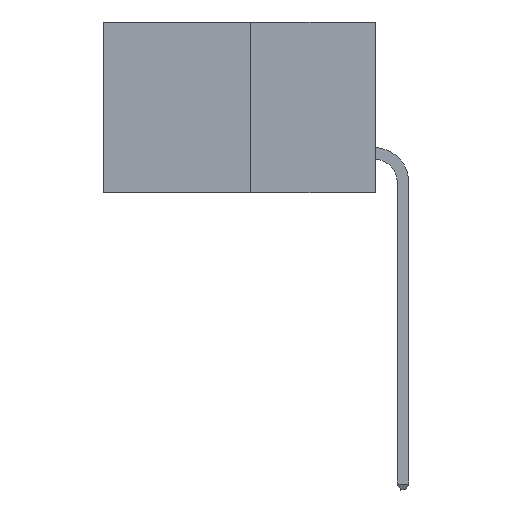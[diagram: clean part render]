
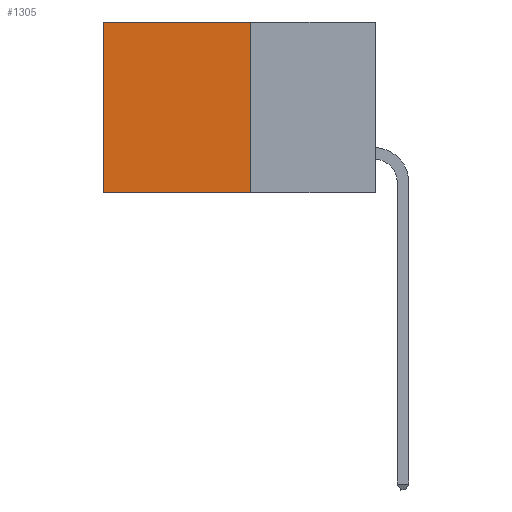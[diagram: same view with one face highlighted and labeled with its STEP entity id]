
A CAD part, left-side view. The second image highlights one B-rep face of the part: STEP entity #1305.
In plain terms, the highlighted planar face has unit normal (-1, 0, 0).
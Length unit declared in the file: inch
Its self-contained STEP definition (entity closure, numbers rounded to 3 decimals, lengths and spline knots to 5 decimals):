
#462 = DIRECTION ( 'NONE',  ( 0., 0., -1. ) ) ;
#862 = CARTESIAN_POINT ( 'NONE',  ( 0.277, 0.59, -0.37 ) ) ;
#1059 = DIRECTION ( 'NONE',  ( 0., 1., 0. ) ) ;
#1109 = CARTESIAN_POINT ( 'NONE',  ( 0.277, 0.27, 0. ) ) ;
#1305 = ADVANCED_FACE ( 'NONE', ( #2072 ), #2721, .F. ) ;
#1325 = AXIS2_PLACEMENT_3D ( 'NONE', #8210, #8078, #462 ) ;
#1344 = ORIENTED_EDGE ( 'NONE', *, *, #5287, .T. ) ;
#1540 = LINE ( 'NONE', #4005, #2067 ) ;
#2067 = VECTOR ( 'NONE', #3599, 39.37008 ) ;
#2072 = FACE_OUTER_BOUND ( 'NONE', #3001, .T. ) ;
#2721 = PLANE ( 'NONE',  #1325 ) ;
#3001 = EDGE_LOOP ( 'NONE', ( #1344, #3753, #3995, #10157 ) ) ;
#3009 = DIRECTION ( 'NONE',  ( 0., 1., 0. ) ) ;
#3547 = VECTOR ( 'NONE', #3009, 39.37008 ) ;
#3599 = DIRECTION ( 'NONE',  ( 0., 0., -1. ) ) ;
#3649 = VERTEX_POINT ( 'NONE', #7518 ) ;
#3675 = LINE ( 'NONE', #9592, #7589 ) ;
#3753 = ORIENTED_EDGE ( 'NONE', *, *, #3822, .F. ) ;
#3822 = EDGE_CURVE ( 'NONE', #8912, #4554, #7713, .T. ) ;
#3995 = ORIENTED_EDGE ( 'NONE', *, *, #7471, .F. ) ;
#4005 = CARTESIAN_POINT ( 'NONE',  ( 0.277, 0.59, -0.37 ) ) ;
#4554 = VERTEX_POINT ( 'NONE', #862 ) ;
#5287 = EDGE_CURVE ( 'NONE', #9945, #4554, #1540, .T. ) ;
#5806 = CARTESIAN_POINT ( 'NONE',  ( 0.277, 0.59, 0. ) ) ;
#6238 = CARTESIAN_POINT ( 'NONE',  ( 0.277, 0.27, -0.37 ) ) ;
#6683 = VECTOR ( 'NONE', #1059, 39.37008 ) ;
#7205 = LINE ( 'NONE', #1109, #6683 ) ;
#7471 = EDGE_CURVE ( 'NONE', #3649, #8912, #3675, .T. ) ;
#7518 = CARTESIAN_POINT ( 'NONE',  ( 0.277, 0.27, 0. ) ) ;
#7589 = VECTOR ( 'NONE', #9639, 39.37008 ) ;
#7713 = LINE ( 'NONE', #6238, #3547 ) ;
#8078 = DIRECTION ( 'NONE',  ( 1., 0., 0. ) ) ;
#8210 = CARTESIAN_POINT ( 'NONE',  ( 0.277, 0.27, -0.37 ) ) ;
#8559 = EDGE_CURVE ( 'NONE', #3649, #9945, #7205, .T. ) ;
#8912 = VERTEX_POINT ( 'NONE', #8996 ) ;
#8996 = CARTESIAN_POINT ( 'NONE',  ( 0.277, 0.27, -0.37 ) ) ;
#9592 = CARTESIAN_POINT ( 'NONE',  ( 0.277, 0.27, -0.37 ) ) ;
#9639 = DIRECTION ( 'NONE',  ( 0., 0., -1. ) ) ;
#9945 = VERTEX_POINT ( 'NONE', #5806 ) ;
#10157 = ORIENTED_EDGE ( 'NONE', *, *, #8559, .T. ) ;
